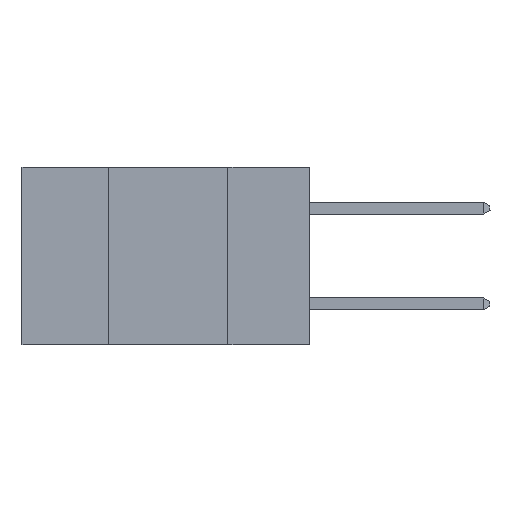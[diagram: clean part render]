
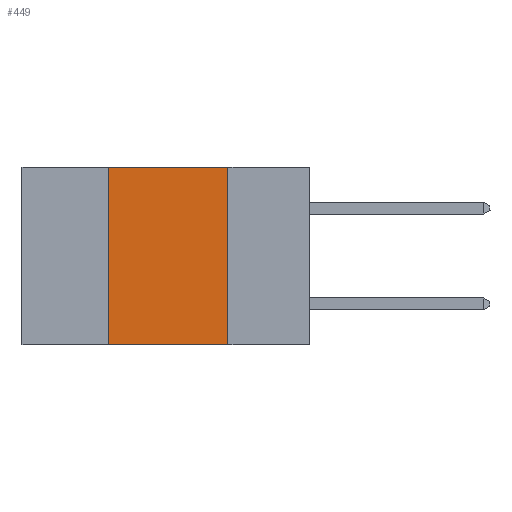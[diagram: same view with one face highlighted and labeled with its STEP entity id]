
A CAD part, left-side view. The second image highlights one B-rep face of the part: STEP entity #449.
In plain terms, the highlighted planar face has unit normal (-1, 0, 0).
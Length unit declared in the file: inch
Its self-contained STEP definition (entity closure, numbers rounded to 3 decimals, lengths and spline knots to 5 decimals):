
#268 = LINE ( 'NONE', #2700, #2034 ) ;
#449 = ADVANCED_FACE ( 'NONE', ( #3564 ), #9753, .F. ) ;
#1184 = CARTESIAN_POINT ( 'NONE',  ( 0., 0.42, 0. ) ) ;
#1722 = DIRECTION ( 'NONE',  ( 0., -1., 0. ) ) ;
#2018 = DIRECTION ( 'NONE',  ( 0., 0., 1. ) ) ;
#2034 = VECTOR ( 'NONE', #1722, 39.37008 ) ;
#2047 = EDGE_CURVE ( 'NONE', #6506, #5946, #8219, .T. ) ;
#2166 = VECTOR ( 'NONE', #7391, 39.37008 ) ;
#2285 = CARTESIAN_POINT ( 'NONE',  ( 0., 0.42, 0. ) ) ;
#2461 = CARTESIAN_POINT ( 'NONE',  ( 0., 0.42, -0.37 ) ) ;
#2472 = VERTEX_POINT ( 'NONE', #10023 ) ;
#2649 = DIRECTION ( 'NONE',  ( 0., 0., -1. ) ) ;
#2700 = CARTESIAN_POINT ( 'NONE',  ( 0., 0.6, 0. ) ) ;
#2719 = ORIENTED_EDGE ( 'NONE', *, *, #5963, .T. ) ;
#3244 = EDGE_CURVE ( 'NONE', #5946, #7201, #268, .T. ) ;
#3564 = FACE_OUTER_BOUND ( 'NONE', #4999, .T. ) ;
#3649 = VECTOR ( 'NONE', #4526, 39.37008 ) ;
#3896 = ORIENTED_EDGE ( 'NONE', *, *, #3244, .F. ) ;
#4526 = DIRECTION ( 'NONE',  ( 0., -1., 0. ) ) ;
#4813 = ORIENTED_EDGE ( 'NONE', *, *, #4990, .F. ) ;
#4990 = EDGE_CURVE ( 'NONE', #7201, #2472, #9823, .T. ) ;
#4999 = EDGE_LOOP ( 'NONE', ( #4813, #3896, #5749, #2719 ) ) ;
#5104 = CARTESIAN_POINT ( 'NONE',  ( 0., 0.6, 0. ) ) ;
#5749 = ORIENTED_EDGE ( 'NONE', *, *, #2047, .F. ) ;
#5946 = VERTEX_POINT ( 'NONE', #2285 ) ;
#5963 = EDGE_CURVE ( 'NONE', #6506, #2472, #9394, .T. ) ;
#6506 = VERTEX_POINT ( 'NONE', #2461 ) ;
#7201 = VERTEX_POINT ( 'NONE', #9830 ) ;
#7391 = DIRECTION ( 'NONE',  ( 0., 0., -1. ) ) ;
#8038 = AXIS2_PLACEMENT_3D ( 'NONE', #5104, #8235, #2649 ) ;
#8219 = LINE ( 'NONE', #1184, #8242 ) ;
#8235 = DIRECTION ( 'NONE',  ( 1., 0., 0. ) ) ;
#8242 = VECTOR ( 'NONE', #2018, 39.37008 ) ;
#9086 = CARTESIAN_POINT ( 'NONE',  ( 0., 0.17, 0. ) ) ;
#9273 = CARTESIAN_POINT ( 'NONE',  ( 0., 0.6, -0.37 ) ) ;
#9394 = LINE ( 'NONE', #9273, #3649 ) ;
#9753 = PLANE ( 'NONE',  #8038 ) ;
#9823 = LINE ( 'NONE', #9086, #2166 ) ;
#9830 = CARTESIAN_POINT ( 'NONE',  ( 0., 0.17, 0. ) ) ;
#10023 = CARTESIAN_POINT ( 'NONE',  ( 0., 0.17, -0.37 ) ) ;
